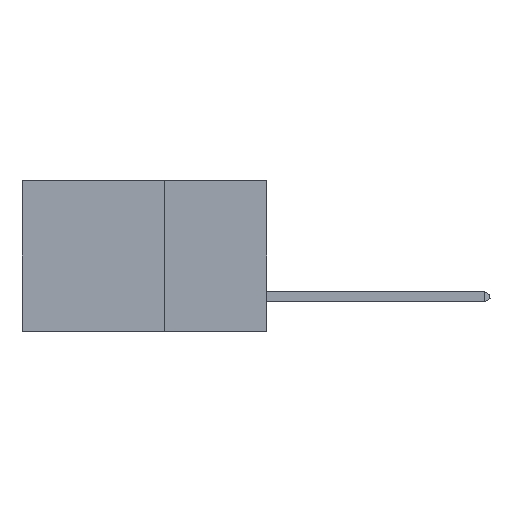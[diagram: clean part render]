
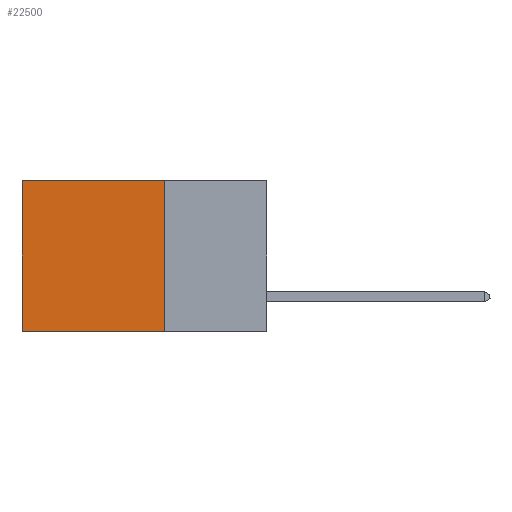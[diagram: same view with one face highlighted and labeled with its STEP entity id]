
A CAD part, left-side view. The second image highlights one B-rep face of the part: STEP entity #22500.
In plain terms, the highlighted planar face has unit normal (-1, 0, 0).
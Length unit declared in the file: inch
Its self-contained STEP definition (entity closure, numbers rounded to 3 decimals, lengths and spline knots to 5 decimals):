
#489 = VECTOR ( 'NONE', #22349, 39.37008 ) ;
#1849 = VECTOR ( 'NONE', #20804, 39.37008 ) ;
#1889 = VERTEX_POINT ( 'NONE', #27597 ) ;
#2335 = CARTESIAN_POINT ( 'NONE',  ( 0.2875, 0.6, 0. ) ) ;
#2750 = EDGE_LOOP ( 'NONE', ( #11404, #11266, #14163, #3547 ) ) ;
#3547 = ORIENTED_EDGE ( 'NONE', *, *, #28638, .T. ) ;
#4492 = VERTEX_POINT ( 'NONE', #12782 ) ;
#4997 = DIRECTION ( 'NONE',  ( 1., 0., 0. ) ) ;
#6057 = AXIS2_PLACEMENT_3D ( 'NONE', #19261, #4997, #27942 ) ;
#7472 = EDGE_CURVE ( 'NONE', #1889, #23533, #19929, .T. ) ;
#9347 = LINE ( 'NONE', #13993, #31351 ) ;
#10043 = FACE_OUTER_BOUND ( 'NONE', #2750, .T. ) ;
#11266 = ORIENTED_EDGE ( 'NONE', *, *, #13879, .F. ) ;
#11404 = ORIENTED_EDGE ( 'NONE', *, *, #17748, .T. ) ;
#11871 = VECTOR ( 'NONE', #15133, 39.37008 ) ;
#12782 = CARTESIAN_POINT ( 'NONE',  ( 0.2875, 0.6, -0.37 ) ) ;
#12895 = CARTESIAN_POINT ( 'NONE',  ( 0.2875, 0.6, 0. ) ) ;
#13879 = EDGE_CURVE ( 'NONE', #23533, #4492, #34998, .T. ) ;
#13993 = CARTESIAN_POINT ( 'NONE',  ( 0.2875, 0.25, 0. ) ) ;
#14163 = ORIENTED_EDGE ( 'NONE', *, *, #7472, .F. ) ;
#15133 = DIRECTION ( 'NONE',  ( 0., 0., -1. ) ) ;
#16855 = DIRECTION ( 'NONE',  ( 0., 1., 0. ) ) ;
#17748 = EDGE_CURVE ( 'NONE', #22436, #4492, #18450, .T. ) ;
#18450 = LINE ( 'NONE', #2335, #489 ) ;
#19261 = CARTESIAN_POINT ( 'NONE',  ( 0.2875, 0.25, 0. ) ) ;
#19929 = LINE ( 'NONE', #26814, #11871 ) ;
#20804 = DIRECTION ( 'NONE',  ( 0., 1., 0. ) ) ;
#22349 = DIRECTION ( 'NONE',  ( 0., 0., -1. ) ) ;
#22436 = VERTEX_POINT ( 'NONE', #12895 ) ;
#22500 = ADVANCED_FACE ( 'NONE', ( #10043 ), #27432, .F. ) ;
#23533 = VERTEX_POINT ( 'NONE', #34789 ) ;
#26814 = CARTESIAN_POINT ( 'NONE',  ( 0.2875, 0.25, 0. ) ) ;
#27432 = PLANE ( 'NONE',  #6057 ) ;
#27597 = CARTESIAN_POINT ( 'NONE',  ( 0.2875, 0.25, 0. ) ) ;
#27942 = DIRECTION ( 'NONE',  ( 0., 0., -1. ) ) ;
#28638 = EDGE_CURVE ( 'NONE', #1889, #22436, #9347, .T. ) ;
#28971 = CARTESIAN_POINT ( 'NONE',  ( 0.2875, 0.25, -0.37 ) ) ;
#31351 = VECTOR ( 'NONE', #16855, 39.37008 ) ;
#34789 = CARTESIAN_POINT ( 'NONE',  ( 0.2875, 0.25, -0.37 ) ) ;
#34998 = LINE ( 'NONE', #28971, #1849 ) ;
